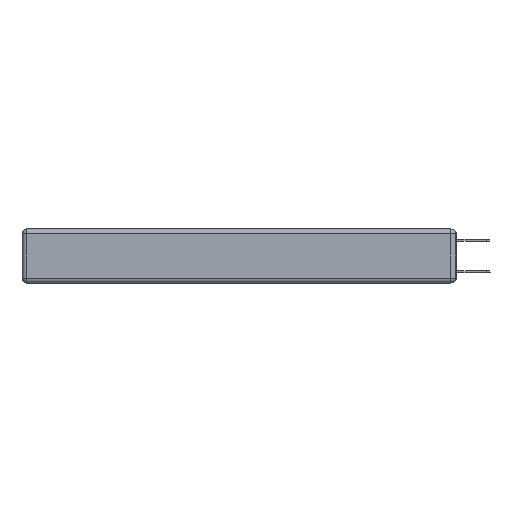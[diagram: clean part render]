
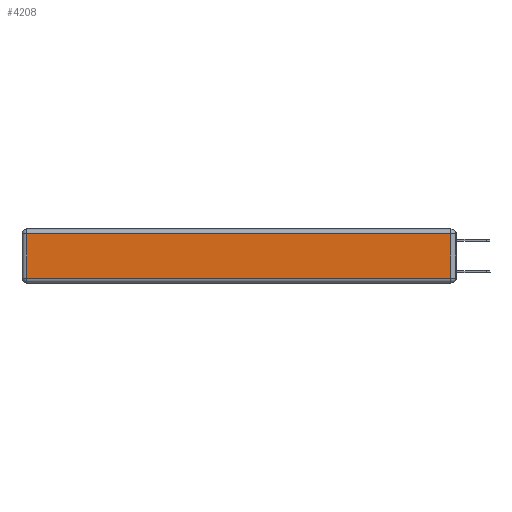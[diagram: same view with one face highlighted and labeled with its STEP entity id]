
A CAD part, left-side view. The second image highlights one B-rep face of the part: STEP entity #4208.
In plain terms, the highlighted planar face has unit normal (-1, 0, 0).
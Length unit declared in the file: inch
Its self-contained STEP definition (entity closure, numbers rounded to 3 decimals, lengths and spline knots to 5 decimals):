
#516 = DIRECTION ( 'NONE',  ( -1., 0., 0. ) ) ;
#1544 = CARTESIAN_POINT ( 'NONE',  ( 0., 0.03, -0.03 ) ) ;
#1585 = VERTEX_POINT ( 'NONE', #5534 ) ;
#1789 = VERTEX_POINT ( 'NONE', #1544 ) ;
#2030 = ORIENTED_EDGE ( 'NONE', *, *, #5080, .T. ) ;
#2281 = LINE ( 'NONE', #4931, #4788 ) ;
#3115 = CARTESIAN_POINT ( 'NONE',  ( 0., 2.75, -0.03 ) ) ;
#3306 = ORIENTED_EDGE ( 'NONE', *, *, #7662, .T. ) ;
#3854 = DIRECTION ( 'NONE',  ( 0., 0., -1. ) ) ;
#4118 = ORIENTED_EDGE ( 'NONE', *, *, #12912, .T. ) ;
#4208 = ADVANCED_FACE ( 'NONE', ( #11865 ), #10456, .T. ) ;
#4209 = CARTESIAN_POINT ( 'NONE',  ( 0., 0.03, -0.313 ) ) ;
#4490 = LINE ( 'NONE', #6976, #8190 ) ;
#4788 = VECTOR ( 'NONE', #3854, 39.37008 ) ;
#4931 = CARTESIAN_POINT ( 'NONE',  ( 0., 2.72, -0.343 ) ) ;
#5080 = EDGE_CURVE ( 'NONE', #8516, #1789, #13691, .T. ) ;
#5408 = DIRECTION ( 'NONE',  ( 0., 0., 1. ) ) ;
#5534 = CARTESIAN_POINT ( 'NONE',  ( 0., 2.72, -0.313 ) ) ;
#6976 = CARTESIAN_POINT ( 'NONE',  ( 0., 0., -0.313 ) ) ;
#7424 = CARTESIAN_POINT ( 'NONE',  ( 0., 2.72, -0.03 ) ) ;
#7523 = VERTEX_POINT ( 'NONE', #7424 ) ;
#7662 = EDGE_CURVE ( 'NONE', #1789, #7523, #11894, .T. ) ;
#8138 = CARTESIAN_POINT ( 'NONE',  ( 0., 0., -0.343 ) ) ;
#8190 = VECTOR ( 'NONE', #12037, 39.37008 ) ;
#8227 = EDGE_CURVE ( 'NONE', #1585, #8516, #4490, .T. ) ;
#8516 = VERTEX_POINT ( 'NONE', #4209 ) ;
#9514 = VECTOR ( 'NONE', #10815, 39.37008 ) ;
#10267 = VECTOR ( 'NONE', #10722, 39.37008 ) ;
#10456 = PLANE ( 'NONE',  #13917 ) ;
#10722 = DIRECTION ( 'NONE',  ( 0., 1., 0. ) ) ;
#10815 = DIRECTION ( 'NONE',  ( 0., 0., 1. ) ) ;
#11216 = CARTESIAN_POINT ( 'NONE',  ( 0., 0.03, -0.343 ) ) ;
#11865 = FACE_OUTER_BOUND ( 'NONE', #16153, .T. ) ;
#11894 = LINE ( 'NONE', #3115, #10267 ) ;
#12037 = DIRECTION ( 'NONE',  ( 0., -1., 0. ) ) ;
#12912 = EDGE_CURVE ( 'NONE', #7523, #1585, #2281, .T. ) ;
#13354 = ORIENTED_EDGE ( 'NONE', *, *, #8227, .T. ) ;
#13691 = LINE ( 'NONE', #11216, #9514 ) ;
#13917 = AXIS2_PLACEMENT_3D ( 'NONE', #8138, #516, #5408 ) ;
#16153 = EDGE_LOOP ( 'NONE', ( #13354, #2030, #3306, #4118 ) ) ;
